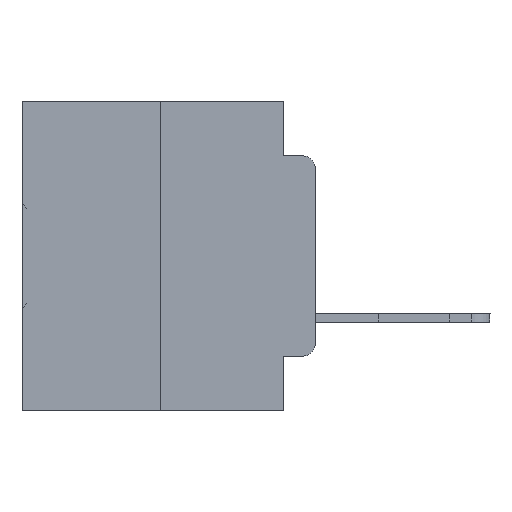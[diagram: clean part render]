
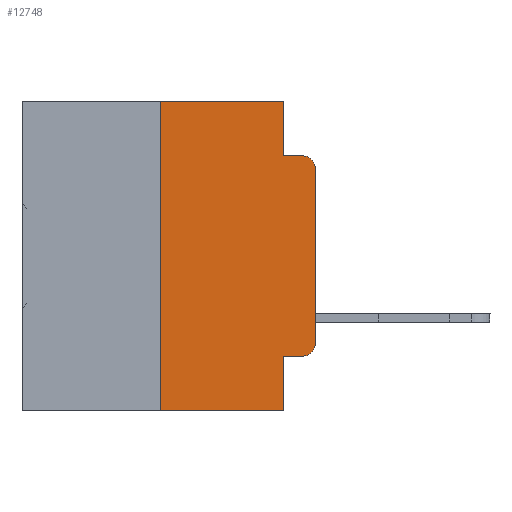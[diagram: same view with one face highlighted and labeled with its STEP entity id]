
A CAD part, left-side view. The second image highlights one B-rep face of the part: STEP entity #12748.
In plain terms, the highlighted planar face has unit normal (-1, 0, 0).
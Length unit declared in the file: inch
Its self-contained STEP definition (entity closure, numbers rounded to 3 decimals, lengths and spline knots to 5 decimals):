
#637 = VECTOR ( 'NONE', #15699, 39.37008 ) ;
#755 = ORIENTED_EDGE ( 'NONE', *, *, #5472, .F. ) ;
#1029 = VERTEX_POINT ( 'NONE', #2708 ) ;
#1680 = ORIENTED_EDGE ( 'NONE', *, *, #32978, .T. ) ;
#2133 = VERTEX_POINT ( 'NONE', #25358 ) ;
#2235 = LINE ( 'NONE', #12923, #11382 ) ;
#2409 = DIRECTION ( 'NONE',  ( 0., 0., -1. ) ) ;
#2708 = CARTESIAN_POINT ( 'NONE',  ( 0., 0., -0.3915 ) ) ;
#3750 = LINE ( 'NONE', #19477, #9445 ) ;
#4056 = AXIS2_PLACEMENT_3D ( 'NONE', #9999, #22515, #24733 ) ;
#4224 = CARTESIAN_POINT ( 'NONE',  ( 0., 0.25, -0.5 ) ) ;
#4415 = VECTOR ( 'NONE', #30882, 39.37008 ) ;
#4447 = EDGE_CURVE ( 'NONE', #1029, #2133, #7994, .T. ) ;
#4772 = ORIENTED_EDGE ( 'NONE', *, *, #32888, .F. ) ;
#5066 = VERTEX_POINT ( 'NONE', #17859 ) ;
#5472 = EDGE_CURVE ( 'NONE', #24493, #17774, #2235, .T. ) ;
#5483 = DIRECTION ( 'NONE',  ( 0., 0., -1. ) ) ;
#5774 = ORIENTED_EDGE ( 'NONE', *, *, #30518, .T. ) ;
#5850 = VERTEX_POINT ( 'NONE', #24592 ) ;
#6528 = DIRECTION ( 'NONE',  ( 1., 0., 0. ) ) ;
#7807 = CIRCLE ( 'NONE', #4056, 0.02 ) ;
#7857 = CARTESIAN_POINT ( 'NONE',  ( 0., 0.051, 0. ) ) ;
#7994 = LINE ( 'NONE', #18319, #21533 ) ;
#8462 = CARTESIAN_POINT ( 'NONE',  ( 0., 0.25, 0. ) ) ;
#8512 = CARTESIAN_POINT ( 'NONE',  ( 0., 0.051, -0.0885 ) ) ;
#9445 = VECTOR ( 'NONE', #14091, 39.37008 ) ;
#9999 = CARTESIAN_POINT ( 'NONE',  ( 0., 0.02, -0.1085 ) ) ;
#10023 = VECTOR ( 'NONE', #25743, 39.37008 ) ;
#10406 = LINE ( 'NONE', #7857, #10873 ) ;
#10873 = VECTOR ( 'NONE', #5483, 39.37008 ) ;
#11382 = VECTOR ( 'NONE', #2409, 39.37008 ) ;
#11478 = VECTOR ( 'NONE', #26874, 39.37008 ) ;
#12748 = ADVANCED_FACE ( 'NONE', ( #30227 ), #17351, .F. ) ;
#12923 = CARTESIAN_POINT ( 'NONE',  ( 0., 0.051, 0. ) ) ;
#14091 = DIRECTION ( 'NONE',  ( 0., -1., 0. ) ) ;
#14268 = ORIENTED_EDGE ( 'NONE', *, *, #16521, .T. ) ;
#14502 = EDGE_CURVE ( 'NONE', #5850, #30030, #10406, .T. ) ;
#15091 = CARTESIAN_POINT ( 'NONE',  ( 0., 0.02, -0.3915 ) ) ;
#15618 = EDGE_CURVE ( 'NONE', #27587, #27405, #32945, .T. ) ;
#15699 = DIRECTION ( 'NONE',  ( 0., -1., 0. ) ) ;
#16045 = CARTESIAN_POINT ( 'NONE',  ( 0., 0.051, -0.4115 ) ) ;
#16224 = AXIS2_PLACEMENT_3D ( 'NONE', #17515, #6528, #20043 ) ;
#16465 = DIRECTION ( 'NONE',  ( 0., 0., 1. ) ) ;
#16521 = EDGE_CURVE ( 'NONE', #24493, #33471, #31620, .T. ) ;
#17290 = DIRECTION ( 'NONE',  ( 0., 0., -1. ) ) ;
#17351 = PLANE ( 'NONE',  #16224 ) ;
#17515 = CARTESIAN_POINT ( 'NONE',  ( 0., 0.473, 0. ) ) ;
#17774 = VERTEX_POINT ( 'NONE', #20638 ) ;
#17859 = CARTESIAN_POINT ( 'NONE',  ( 0., 0.02, -0.0885 ) ) ;
#18319 = CARTESIAN_POINT ( 'NONE',  ( 0., 0., 0. ) ) ;
#18390 = LINE ( 'NONE', #26185, #637 ) ;
#18735 = EDGE_CURVE ( 'NONE', #33471, #1029, #27467, .T. ) ;
#19477 = CARTESIAN_POINT ( 'NONE',  ( 0., 0.051, -0.0885 ) ) ;
#20043 = DIRECTION ( 'NONE',  ( 0., 0., -1. ) ) ;
#20053 = CARTESIAN_POINT ( 'NONE',  ( 0., 0.25, 0. ) ) ;
#20192 = ORIENTED_EDGE ( 'NONE', *, *, #4447, .T. ) ;
#20638 = CARTESIAN_POINT ( 'NONE',  ( 0., 0.051, -0.5 ) ) ;
#21533 = VECTOR ( 'NONE', #16465, 39.37008 ) ;
#22515 = DIRECTION ( 'NONE',  ( -1., 0., 0. ) ) ;
#22756 = ORIENTED_EDGE ( 'NONE', *, *, #24085, .F. ) ;
#24085 = EDGE_CURVE ( 'NONE', #27405, #5850, #27962, .T. ) ;
#24331 = EDGE_LOOP ( 'NONE', ( #20192, #1680, #4772, #24953, #22756, #28683, #5774, #755, #14268, #26599 ) ) ;
#24493 = VERTEX_POINT ( 'NONE', #30948 ) ;
#24592 = CARTESIAN_POINT ( 'NONE',  ( 0., 0.051, 0. ) ) ;
#24733 = DIRECTION ( 'NONE',  ( 0., 0., -1. ) ) ;
#24750 = AXIS2_PLACEMENT_3D ( 'NONE', #15091, #27955, #17290 ) ;
#24953 = ORIENTED_EDGE ( 'NONE', *, *, #14502, .F. ) ;
#25358 = CARTESIAN_POINT ( 'NONE',  ( 0., 0., -0.1085 ) ) ;
#25743 = DIRECTION ( 'NONE',  ( 0., -1., 0. ) ) ;
#26077 = CARTESIAN_POINT ( 'NONE',  ( 0., 0.473, 0. ) ) ;
#26185 = CARTESIAN_POINT ( 'NONE',  ( 0., 0.473, -0.5 ) ) ;
#26599 = ORIENTED_EDGE ( 'NONE', *, *, #18735, .T. ) ;
#26874 = DIRECTION ( 'NONE',  ( 0., -1., 0. ) ) ;
#27405 = VERTEX_POINT ( 'NONE', #8462 ) ;
#27416 = CARTESIAN_POINT ( 'NONE',  ( 0., 0.02, -0.4115 ) ) ;
#27467 = CIRCLE ( 'NONE', #24750, 0.02 ) ;
#27587 = VERTEX_POINT ( 'NONE', #4224 ) ;
#27955 = DIRECTION ( 'NONE',  ( -1., 0., 0. ) ) ;
#27962 = LINE ( 'NONE', #26077, #10023 ) ;
#28683 = ORIENTED_EDGE ( 'NONE', *, *, #15618, .F. ) ;
#30030 = VERTEX_POINT ( 'NONE', #8512 ) ;
#30227 = FACE_OUTER_BOUND ( 'NONE', #24331, .T. ) ;
#30518 = EDGE_CURVE ( 'NONE', #27587, #17774, #18390, .T. ) ;
#30882 = DIRECTION ( 'NONE',  ( 0., 0., 1. ) ) ;
#30948 = CARTESIAN_POINT ( 'NONE',  ( 0., 0.051, -0.4115 ) ) ;
#31620 = LINE ( 'NONE', #16045, #11478 ) ;
#32888 = EDGE_CURVE ( 'NONE', #30030, #5066, #3750, .T. ) ;
#32945 = LINE ( 'NONE', #20053, #4415 ) ;
#32978 = EDGE_CURVE ( 'NONE', #2133, #5066, #7807, .T. ) ;
#33471 = VERTEX_POINT ( 'NONE', #27416 ) ;
